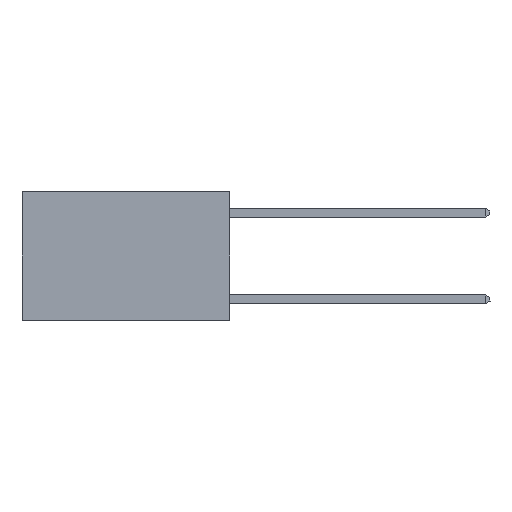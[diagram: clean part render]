
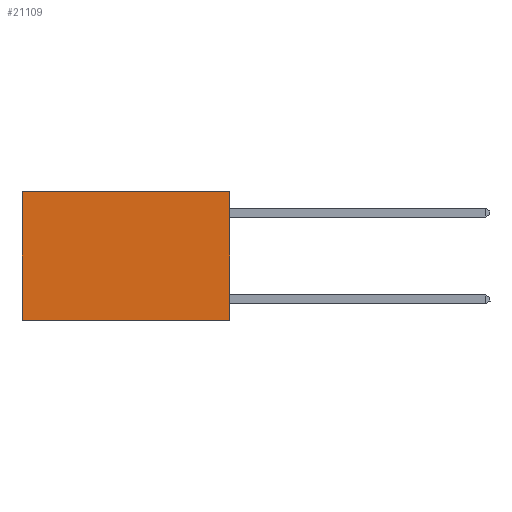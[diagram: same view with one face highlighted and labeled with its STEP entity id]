
A CAD part, left-side view. The second image highlights one B-rep face of the part: STEP entity #21109.
In plain terms, the highlighted planar face has unit normal (-1, 0, 0).
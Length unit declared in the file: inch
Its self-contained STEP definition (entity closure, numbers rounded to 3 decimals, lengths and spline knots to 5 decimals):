
#256 = VECTOR ( 'NONE', #15611, 39.37008 ) ;
#272 = ORIENTED_EDGE ( 'NONE', *, *, #6988, .F. ) ;
#1264 = DIRECTION ( 'NONE',  ( 0., 1., 0. ) ) ;
#2391 = CARTESIAN_POINT ( 'NONE',  ( 0.2625, 0., 0. ) ) ;
#2523 = LINE ( 'NONE', #6979, #256 ) ;
#3000 = LINE ( 'NONE', #10545, #17465 ) ;
#4065 = VERTEX_POINT ( 'NONE', #2391 ) ;
#6979 = CARTESIAN_POINT ( 'NONE',  ( 0.2625, 0.6, 0. ) ) ;
#6988 = EDGE_CURVE ( 'NONE', #18787, #19503, #14007, .T. ) ;
#7921 = CARTESIAN_POINT ( 'NONE',  ( 0.2625, 0.6, -0.37 ) ) ;
#8505 = DIRECTION ( 'NONE',  ( 0., 0., -1. ) ) ;
#9118 = VECTOR ( 'NONE', #25353, 39.37008 ) ;
#10545 = CARTESIAN_POINT ( 'NONE',  ( 0.2625, 0., 0. ) ) ;
#11014 = CARTESIAN_POINT ( 'NONE',  ( 0.2625, 0., 0. ) ) ;
#12698 = DIRECTION ( 'NONE',  ( 1., 0., 0. ) ) ;
#13162 = EDGE_CURVE ( 'NONE', #4065, #18787, #3000, .T. ) ;
#13632 = CARTESIAN_POINT ( 'NONE',  ( 0.2625, 0.6, 0. ) ) ;
#14007 = LINE ( 'NONE', #19625, #22725 ) ;
#14449 = PLANE ( 'NONE',  #19221 ) ;
#14899 = LINE ( 'NONE', #11014, #9118 ) ;
#15611 = DIRECTION ( 'NONE',  ( 0., 0., -1. ) ) ;
#16708 = EDGE_CURVE ( 'NONE', #25192, #19503, #2523, .T. ) ;
#16843 = DIRECTION ( 'NONE',  ( 0., 0., -1. ) ) ;
#17465 = VECTOR ( 'NONE', #16843, 39.37008 ) ;
#17643 = ORIENTED_EDGE ( 'NONE', *, *, #13162, .F. ) ;
#18787 = VERTEX_POINT ( 'NONE', #19781 ) ;
#19221 = AXIS2_PLACEMENT_3D ( 'NONE', #25009, #12698, #8505 ) ;
#19503 = VERTEX_POINT ( 'NONE', #7921 ) ;
#19625 = CARTESIAN_POINT ( 'NONE',  ( 0.2625, 0., -0.37 ) ) ;
#19781 = CARTESIAN_POINT ( 'NONE',  ( 0.2625, 0., -0.37 ) ) ;
#20948 = FACE_OUTER_BOUND ( 'NONE', #22973, .T. ) ;
#21109 = ADVANCED_FACE ( 'NONE', ( #20948 ), #14449, .F. ) ;
#22725 = VECTOR ( 'NONE', #1264, 39.37008 ) ;
#22973 = EDGE_LOOP ( 'NONE', ( #23753, #272, #17643, #26159 ) ) ;
#23753 = ORIENTED_EDGE ( 'NONE', *, *, #16708, .T. ) ;
#25009 = CARTESIAN_POINT ( 'NONE',  ( 0.2625, 0., 0. ) ) ;
#25192 = VERTEX_POINT ( 'NONE', #13632 ) ;
#25353 = DIRECTION ( 'NONE',  ( 0., 1., 0. ) ) ;
#25704 = EDGE_CURVE ( 'NONE', #4065, #25192, #14899, .T. ) ;
#26159 = ORIENTED_EDGE ( 'NONE', *, *, #25704, .T. ) ;
